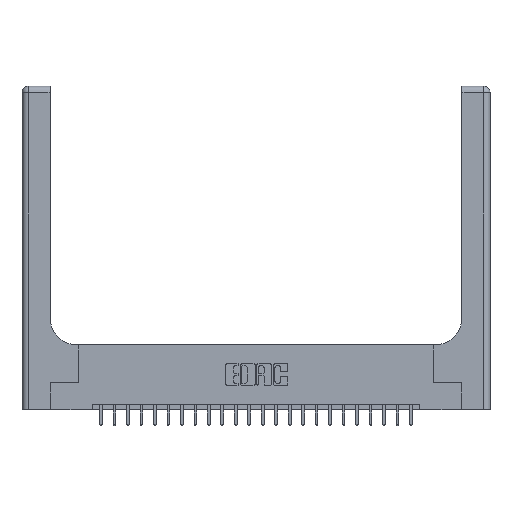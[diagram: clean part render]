
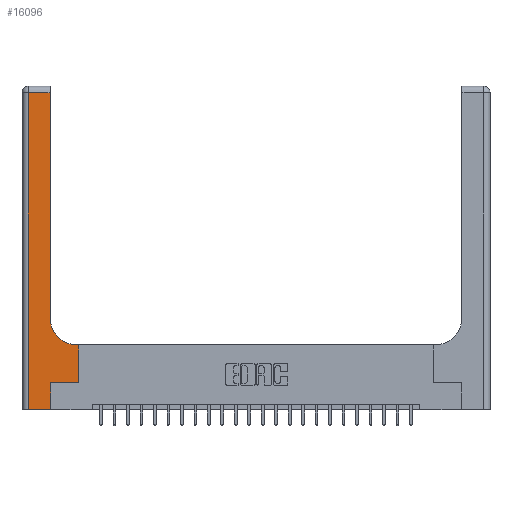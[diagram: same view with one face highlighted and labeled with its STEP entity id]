
A CAD part, top view. The second image highlights one B-rep face of the part: STEP entity #16096.
In plain terms, the highlighted planar face has unit normal (0, 0, 1).
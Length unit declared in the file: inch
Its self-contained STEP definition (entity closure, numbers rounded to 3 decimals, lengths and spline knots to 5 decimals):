
#243 = EDGE_CURVE ( 'NONE', #18764, #6475, #21615, .T. ) ;
#369 = DIRECTION ( 'NONE',  ( -1., 0., 0. ) ) ;
#568 = DIRECTION ( 'NONE',  ( 0., 0., -1. ) ) ;
#676 = CARTESIAN_POINT ( 'NONE',  ( 0.06, 2.94, 0.37 ) ) ;
#900 = CARTESIAN_POINT ( 'NONE',  ( 0.06, 0., 0.37 ) ) ;
#1328 = EDGE_CURVE ( 'NONE', #9177, #4803, #18805, .T. ) ;
#1892 = VECTOR ( 'NONE', #10196, 39.37008 ) ;
#1992 = CARTESIAN_POINT ( 'NONE',  ( 0.265, 0., 0.37 ) ) ;
#2000 = EDGE_CURVE ( 'NONE', #6475, #10695, #9467, .T. ) ;
#2488 = ORIENTED_EDGE ( 'NONE', *, *, #2515, .T. ) ;
#2515 = EDGE_CURVE ( 'NONE', #17115, #13148, #14799, .T. ) ;
#2819 = DIRECTION ( 'NONE',  ( 1., 0., 0. ) ) ;
#2878 = CARTESIAN_POINT ( 'NONE',  ( 0.26, 2.94, 0.37 ) ) ;
#3091 = EDGE_LOOP ( 'NONE', ( #6430, #2488, #21071, #4973, #4952, #22216, #7777, #5721, #23005 ) ) ;
#3878 = CIRCLE ( 'NONE', #15369, 0.25 ) ;
#4017 = EDGE_CURVE ( 'NONE', #13148, #18764, #11056, .T. ) ;
#4771 = CARTESIAN_POINT ( 'NONE',  ( 0.26, 0.6, 0.37 ) ) ;
#4803 = VERTEX_POINT ( 'NONE', #12571 ) ;
#4952 = ORIENTED_EDGE ( 'NONE', *, *, #2000, .T. ) ;
#4973 = ORIENTED_EDGE ( 'NONE', *, *, #243, .T. ) ;
#5172 = VECTOR ( 'NONE', #9637, 39.37008 ) ;
#5721 = ORIENTED_EDGE ( 'NONE', *, *, #1328, .T. ) ;
#5726 = CARTESIAN_POINT ( 'NONE',  ( 0.528, 0.25, 0.37 ) ) ;
#5812 = LINE ( 'NONE', #13078, #11694 ) ;
#6092 = VECTOR ( 'NONE', #11953, 39.37008 ) ;
#6258 = CARTESIAN_POINT ( 'NONE',  ( 0.265, 0.25, 0.37 ) ) ;
#6347 = EDGE_CURVE ( 'NONE', #4803, #14106, #3878, .T. ) ;
#6430 = ORIENTED_EDGE ( 'NONE', *, *, #6800, .T. ) ;
#6475 = VERTEX_POINT ( 'NONE', #6735 ) ;
#6586 = CARTESIAN_POINT ( 'NONE',  ( 0.51, 0.85, 0.37 ) ) ;
#6735 = CARTESIAN_POINT ( 'NONE',  ( 0.265, 0., 0.37 ) ) ;
#6800 = EDGE_CURVE ( 'NONE', #14106, #17115, #9497, .T. ) ;
#7777 = ORIENTED_EDGE ( 'NONE', *, *, #12371, .T. ) ;
#7891 = CARTESIAN_POINT ( 'NONE',  ( 0.265, 0.25, 0.37 ) ) ;
#9177 = VERTEX_POINT ( 'NONE', #15406 ) ;
#9467 = LINE ( 'NONE', #1992, #18489 ) ;
#9497 = LINE ( 'NONE', #22027, #17397 ) ;
#9559 = EDGE_CURVE ( 'NONE', #10695, #22464, #10516, .T. ) ;
#9637 = DIRECTION ( 'NONE',  ( 0., -1., 0. ) ) ;
#10196 = DIRECTION ( 'NONE',  ( -1., 0., 0. ) ) ;
#10516 = LINE ( 'NONE', #7891, #21766 ) ;
#10679 = DIRECTION ( 'NONE',  ( 0., 0., -1. ) ) ;
#10695 = VERTEX_POINT ( 'NONE', #6258 ) ;
#11056 = LINE ( 'NONE', #14831, #5172 ) ;
#11440 = FACE_OUTER_BOUND ( 'NONE', #3091, .T. ) ;
#11694 = VECTOR ( 'NONE', #18590, 39.37008 ) ;
#11789 = CARTESIAN_POINT ( 'NONE',  ( 0., 0., 0.37 ) ) ;
#11953 = DIRECTION ( 'NONE',  ( -1., 0., 0. ) ) ;
#12022 = AXIS2_PLACEMENT_3D ( 'NONE', #14308, #10679, #369 ) ;
#12371 = EDGE_CURVE ( 'NONE', #22464, #9177, #5812, .T. ) ;
#12571 = CARTESIAN_POINT ( 'NONE',  ( 0.51, 0.6, 0.37 ) ) ;
#12913 = DIRECTION ( 'NONE',  ( 0., 1., 0. ) ) ;
#13078 = CARTESIAN_POINT ( 'NONE',  ( 0.528, 0.25, 0.37 ) ) ;
#13148 = VERTEX_POINT ( 'NONE', #676 ) ;
#13171 = DIRECTION ( 'NONE',  ( 1., 0., 0. ) ) ;
#14106 = VERTEX_POINT ( 'NONE', #16855 ) ;
#14308 = CARTESIAN_POINT ( 'NONE',  ( 0., 3., 0.37 ) ) ;
#14799 = LINE ( 'NONE', #22725, #6092 ) ;
#14831 = CARTESIAN_POINT ( 'NONE',  ( 0.06, 3., 0.37 ) ) ;
#15369 = AXIS2_PLACEMENT_3D ( 'NONE', #6586, #568, #13171 ) ;
#15406 = CARTESIAN_POINT ( 'NONE',  ( 0.528, 0.6, 0.37 ) ) ;
#16096 = ADVANCED_FACE ( 'NONE', ( #11440 ), #18423, .F. ) ;
#16855 = CARTESIAN_POINT ( 'NONE',  ( 0.26, 0.85, 0.37 ) ) ;
#17115 = VERTEX_POINT ( 'NONE', #2878 ) ;
#17397 = VECTOR ( 'NONE', #12913, 39.37008 ) ;
#18423 = PLANE ( 'NONE',  #12022 ) ;
#18489 = VECTOR ( 'NONE', #21654, 39.37008 ) ;
#18590 = DIRECTION ( 'NONE',  ( 0., 1., 0. ) ) ;
#18764 = VERTEX_POINT ( 'NONE', #900 ) ;
#18805 = LINE ( 'NONE', #4771, #1892 ) ;
#19395 = VECTOR ( 'NONE', #2819, 39.37008 ) ;
#20441 = DIRECTION ( 'NONE',  ( 1., 0., 0. ) ) ;
#21071 = ORIENTED_EDGE ( 'NONE', *, *, #4017, .T. ) ;
#21615 = LINE ( 'NONE', #11789, #19395 ) ;
#21654 = DIRECTION ( 'NONE',  ( 0., 1., 0. ) ) ;
#21766 = VECTOR ( 'NONE', #20441, 39.37008 ) ;
#22027 = CARTESIAN_POINT ( 'NONE',  ( 0.26, 3., 0.37 ) ) ;
#22216 = ORIENTED_EDGE ( 'NONE', *, *, #9559, .T. ) ;
#22464 = VERTEX_POINT ( 'NONE', #5726 ) ;
#22725 = CARTESIAN_POINT ( 'NONE',  ( 0., 2.94, 0.37 ) ) ;
#23005 = ORIENTED_EDGE ( 'NONE', *, *, #6347, .T. ) ;
